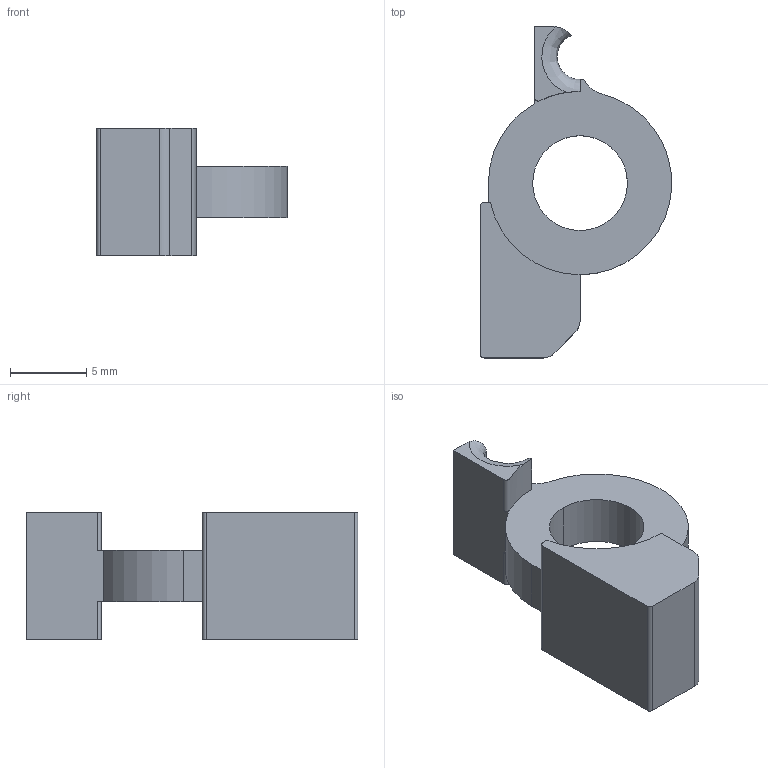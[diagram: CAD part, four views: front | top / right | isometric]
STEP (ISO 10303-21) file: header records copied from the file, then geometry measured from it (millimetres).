
FILE_DESCRIPTION (( 'STEP AP214' ), '1' );
FILE_NAME ('Imura_V2_Sear_Flapper.step', '2015-01-26T00:08:47', ( 'WarFairy' ), ( '' ), 'SwSTEP 2.0', 'SolidWorks 2013', '' );
FILE_SCHEMA (( 'AUTOMOTIVE_DESIGN' ));
Length unit declared in the file: millimetre
Products named in the file (1): Imura_V2_Sear_Flapper
Bounding box: 12.52 x 21.71 x 8.35 mm (x, y, z)
Volume: 720.5 mm3; surface area: 758.9 mm2
Topology: 1 solids, 1 shells, 36 faces, 98 edges, 64 vertices
Faces by surface type: cylinder 18, plane 16, bspline 2
Entity records: 1269 total; most frequent: CARTESIAN_POINT 311, DIRECTION 196, ORIENTED_EDGE 196, EDGE_CURVE 98, AXIS2_PLACEMENT_3D 71, VERTEX_POINT 64, LINE 54, VECTOR 54
